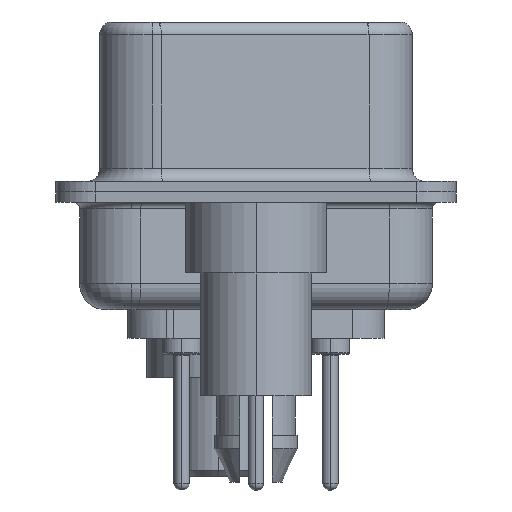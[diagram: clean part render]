
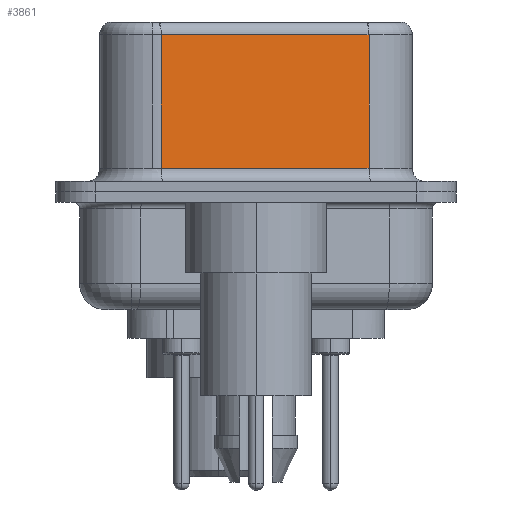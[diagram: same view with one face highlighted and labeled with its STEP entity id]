
A CAD part, left-side view. The second image highlights one B-rep face of the part: STEP entity #3861.
In plain terms, the highlighted planar face has unit normal (-0.985, -0.174, 0).
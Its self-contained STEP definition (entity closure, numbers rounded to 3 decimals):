
#193 = CARTESIAN_POINT ( 'NONE',  ( 5.132, -4.322, 6.52 ) ) ;
#436 = CARTESIAN_POINT ( 'NONE',  ( 3.73, 3.628, 6.02 ) ) ;
#998 = ORIENTED_EDGE ( 'NONE', *, *, #8776, .T. ) ;
#3335 = CARTESIAN_POINT ( 'NONE',  ( 5.132, -4.322, 0.9 ) ) ;
#3383 = VECTOR ( 'NONE', #31273, 1000. ) ;
#3861 = ADVANCED_FACE ( 'NONE', ( #30858 ), #5848, .F. ) ;
#4493 = DIRECTION ( 'NONE',  ( 0., 0., -1. ) ) ;
#5770 = CARTESIAN_POINT ( 'NONE',  ( 5.132, -4.322, 6.02 ) ) ;
#5848 = PLANE ( 'NONE',  #26899 ) ;
#6099 = VECTOR ( 'NONE', #26315, 1000. ) ;
#7581 = LINE ( 'NONE', #3335, #25593 ) ;
#8776 = EDGE_CURVE ( 'NONE', #19453, #21708, #27328, .T. ) ;
#9658 = EDGE_CURVE ( 'NONE', #21708, #18444, #17079, .T. ) ;
#10142 = CARTESIAN_POINT ( 'NONE',  ( 5.132, -4.322, 0.9 ) ) ;
#10816 = EDGE_CURVE ( 'NONE', #19453, #30742, #23903, .T. ) ;
#11707 = EDGE_LOOP ( 'NONE', ( #15370, #998, #21228, #32090 ) ) ;
#13283 = CARTESIAN_POINT ( 'NONE',  ( 5.132, -4.322, 6.52 ) ) ;
#15145 = CARTESIAN_POINT ( 'NONE',  ( 3.73, 3.628, 0.9 ) ) ;
#15370 = ORIENTED_EDGE ( 'NONE', *, *, #10816, .F. ) ;
#17079 = LINE ( 'NONE', #25035, #30044 ) ;
#18444 = VERTEX_POINT ( 'NONE', #15145 ) ;
#19453 = VERTEX_POINT ( 'NONE', #31306 ) ;
#21081 = EDGE_CURVE ( 'NONE', #18444, #30742, #7581, .T. ) ;
#21228 = ORIENTED_EDGE ( 'NONE', *, *, #9658, .T. ) ;
#21708 = VERTEX_POINT ( 'NONE', #436 ) ;
#22862 = DIRECTION ( 'NONE',  ( -0.174, 0.985, 0. ) ) ;
#23809 = DIRECTION ( 'NONE',  ( 0.174, -0.985, 0. ) ) ;
#23903 = LINE ( 'NONE', #13283, #3383 ) ;
#25035 = CARTESIAN_POINT ( 'NONE',  ( 3.73, 3.628, 6.52 ) ) ;
#25593 = VECTOR ( 'NONE', #23809, 1000. ) ;
#26315 = DIRECTION ( 'NONE',  ( -0.174, 0.985, 0. ) ) ;
#26899 = AXIS2_PLACEMENT_3D ( 'NONE', #193, #28318, #22862 ) ;
#27328 = LINE ( 'NONE', #5770, #6099 ) ;
#28318 = DIRECTION ( 'NONE',  ( 0.985, 0.174, 0. ) ) ;
#30044 = VECTOR ( 'NONE', #4493, 1000. ) ;
#30742 = VERTEX_POINT ( 'NONE', #10142 ) ;
#30858 = FACE_OUTER_BOUND ( 'NONE', #11707, .T. ) ;
#31273 = DIRECTION ( 'NONE',  ( 0., 0., -1. ) ) ;
#31306 = CARTESIAN_POINT ( 'NONE',  ( 5.132, -4.322, 6.02 ) ) ;
#32090 = ORIENTED_EDGE ( 'NONE', *, *, #21081, .T. ) ;
